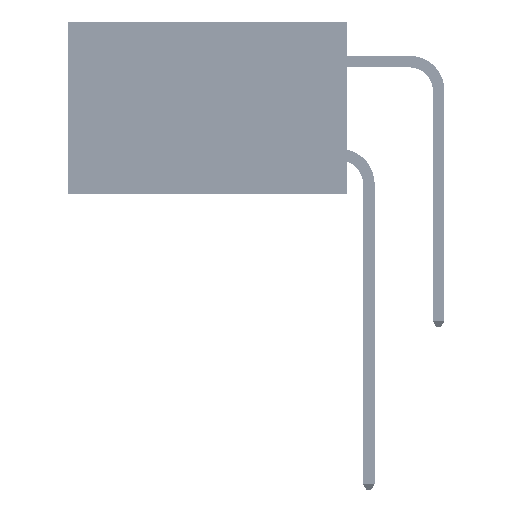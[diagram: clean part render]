
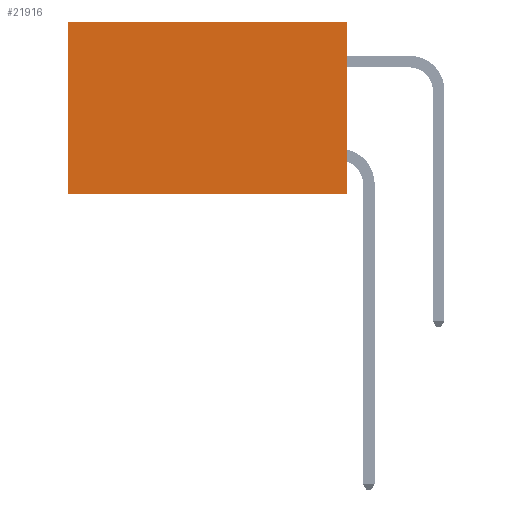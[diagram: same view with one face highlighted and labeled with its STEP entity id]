
A CAD part, left-side view. The second image highlights one B-rep face of the part: STEP entity #21916.
In plain terms, the highlighted planar face has unit normal (-1, 0, 0).
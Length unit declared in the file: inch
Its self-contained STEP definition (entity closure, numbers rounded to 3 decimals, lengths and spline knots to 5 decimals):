
#405 = EDGE_CURVE ( 'NONE', #30471, #13625, #2323, .T. ) ;
#1530 = AXIS2_PLACEMENT_3D ( 'NONE', #23429, #51372, #3178 ) ;
#2323 = LINE ( 'NONE', #45272, #4189 ) ;
#3178 = DIRECTION ( 'NONE',  ( 0., 0., -1. ) ) ;
#3348 = DIRECTION ( 'NONE',  ( 0., 0., -1. ) ) ;
#3657 = LINE ( 'NONE', #35203, #21737 ) ;
#3926 = CARTESIAN_POINT ( 'NONE',  ( 0.2875, 0.6, -0.37 ) ) ;
#4189 = VECTOR ( 'NONE', #49512, 39.37008 ) ;
#7620 = CARTESIAN_POINT ( 'NONE',  ( 0.2875, 0.6, 0. ) ) ;
#10592 = EDGE_CURVE ( 'NONE', #13625, #36889, #44324, .T. ) ;
#13625 = VERTEX_POINT ( 'NONE', #7620 ) ;
#18094 = VECTOR ( 'NONE', #32049, 39.37008 ) ;
#21737 = VECTOR ( 'NONE', #3348, 39.37008 ) ;
#21916 = ADVANCED_FACE ( 'NONE', ( #40890 ), #39086, .F. ) ;
#22690 = CARTESIAN_POINT ( 'NONE',  ( 0.2875, 0., 0. ) ) ;
#23429 = CARTESIAN_POINT ( 'NONE',  ( 0.2875, 0., 0. ) ) ;
#24345 = ORIENTED_EDGE ( 'NONE', *, *, #44290, .F. ) ;
#26011 = ORIENTED_EDGE ( 'NONE', *, *, #10592, .T. ) ;
#28034 = CARTESIAN_POINT ( 'NONE',  ( 0.2875, 0., -0.37 ) ) ;
#28758 = LINE ( 'NONE', #28034, #18094 ) ;
#30471 = VERTEX_POINT ( 'NONE', #22690 ) ;
#32049 = DIRECTION ( 'NONE',  ( 0., 1., 0. ) ) ;
#34980 = DIRECTION ( 'NONE',  ( 0., 0., -1. ) ) ;
#35203 = CARTESIAN_POINT ( 'NONE',  ( 0.2875, 0., 0. ) ) ;
#36801 = VERTEX_POINT ( 'NONE', #43542 ) ;
#36889 = VERTEX_POINT ( 'NONE', #3926 ) ;
#37456 = EDGE_CURVE ( 'NONE', #36801, #36889, #28758, .T. ) ;
#39086 = PLANE ( 'NONE',  #1530 ) ;
#39338 = ORIENTED_EDGE ( 'NONE', *, *, #37456, .F. ) ;
#40890 = FACE_OUTER_BOUND ( 'NONE', #42956, .T. ) ;
#42572 = CARTESIAN_POINT ( 'NONE',  ( 0.2875, 0.6, 0. ) ) ;
#42956 = EDGE_LOOP ( 'NONE', ( #26011, #39338, #24345, #47077 ) ) ;
#43542 = CARTESIAN_POINT ( 'NONE',  ( 0.2875, 0., -0.37 ) ) ;
#43677 = VECTOR ( 'NONE', #34980, 39.37008 ) ;
#44290 = EDGE_CURVE ( 'NONE', #30471, #36801, #3657, .T. ) ;
#44324 = LINE ( 'NONE', #42572, #43677 ) ;
#45272 = CARTESIAN_POINT ( 'NONE',  ( 0.2875, 0., 0. ) ) ;
#47077 = ORIENTED_EDGE ( 'NONE', *, *, #405, .T. ) ;
#49512 = DIRECTION ( 'NONE',  ( 0., 1., 0. ) ) ;
#51372 = DIRECTION ( 'NONE',  ( 1., 0., 0. ) ) ;
